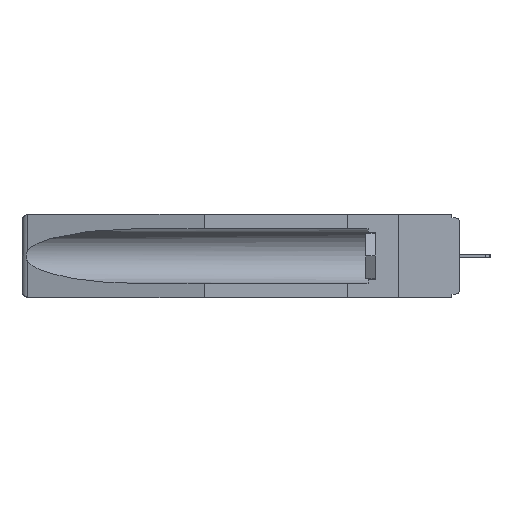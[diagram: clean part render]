
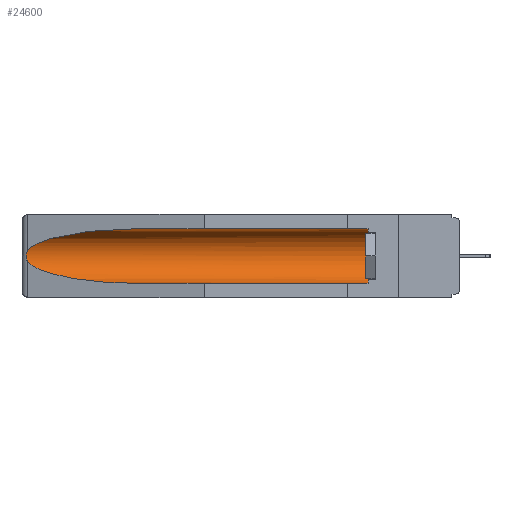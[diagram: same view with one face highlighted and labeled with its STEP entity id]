
A CAD part, left-side view. The second image highlights one B-rep face of the part: STEP entity #24600.
In plain terms, the highlighted cylindrical face has radius 2.857 mm (diameter 5.715 mm), a partial arc.
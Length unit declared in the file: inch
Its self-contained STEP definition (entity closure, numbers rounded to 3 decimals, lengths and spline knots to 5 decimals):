
#1335 = VERTEX_POINT ( 'NONE', #24187 ) ;
#2050 = CARTESIAN_POINT ( 'NONE',  ( 0.155, 1.07973, -0.284 ) ) ;
#2057 = ORIENTED_EDGE ( 'NONE', *, *, #10359, .T. ) ;
#2761 = EDGE_CURVE ( 'NONE', #25303, #18392, #21316, .T. ) ;
#2961 = DIRECTION ( 'NONE',  ( 0., -1., 0. ) ) ;
#3534 = EDGE_CURVE ( 'NONE', #18392, #1335, #25561, .T. ) ;
#4042 = CARTESIAN_POINT ( 'NONE',  ( 0.26597, 1.52961, -0.15275 ) ) ;
#4124 = CARTESIAN_POINT ( 'NONE',  ( 0.21114, 1.30732, -0.284 ) ) ;
#4595 = CARTESIAN_POINT ( 'NONE',  ( 0.2673, 1.53269, -0.17917 ) ) ;
#5179 = CARTESIAN_POINT ( 'NONE',  ( 0.155, 1.07973, -0.059 ) ) ;
#5829 = CYLINDRICAL_SURFACE ( 'NONE', #21166, 0.1125 ) ;
#6156 = CARTESIAN_POINT ( 'NONE',  ( 0.26537, 1.52718, -0.19328 ) ) ;
#6591 = CARTESIAN_POINT ( 'NONE',  ( 0.155, 0.126, -0.284 ) ) ;
#6625 = CARTESIAN_POINT ( 'NONE',  ( 0.26654, 1.53092, -0.15636 ) ) ;
#6821 = CARTESIAN_POINT ( 'NONE',  ( 0.155, -0.30754, -0.284 ) ) ;
#6889 = DIRECTION ( 'NONE',  ( 0., 1., 0. ) ) ;
#7673 = ORIENTED_EDGE ( 'NONE', *, *, #3534, .T. ) ;
#8034 = EDGE_CURVE ( 'NONE', #24053, #15591, #17546, .T. ) ;
#8267 =( BOUNDED_CURVE ( )  B_SPLINE_CURVE ( 3, ( #5179, #26425, #13939, #20240 ),
 .UNSPECIFIED., .F., .T. ) 
 B_SPLINE_CURVE_WITH_KNOTS ( ( 4, 4 ),
 ( 4.71239, 6.08839 ),
 .UNSPECIFIED. ) 
 CURVE ( )  GEOMETRIC_REPRESENTATION_ITEM ( )  RATIONAL_B_SPLINE_CURVE ( ( 1., 0.848, 0.848, 1. ) ) 
 REPRESENTATION_ITEM ( '' )  );
#8889 = CARTESIAN_POINT ( 'NONE',  ( 0.155, 0.126, -0.059 ) ) ;
#10359 = EDGE_CURVE ( 'NONE', #15591, #17185, #16858, .T. ) ;
#10468 = DIRECTION ( 'NONE',  ( 0., 1., 0. ) ) ;
#10754 = CARTESIAN_POINT ( 'NONE',  ( 0.2673, 1.5327, -0.16383 ) ) ;
#10794 = EDGE_CURVE ( 'NONE', #1335, #24053, #8267, .T. ) ;
#11176 = VECTOR ( 'NONE', #22658, 39.37008 ) ;
#11189 = CARTESIAN_POINT ( 'NONE',  ( 0.155, 1.07973, -0.284 ) ) ;
#12402 = CARTESIAN_POINT ( 'NONE',  ( 0.2675, 1.53308, -0.16763 ) ) ;
#12547 = CARTESIAN_POINT ( 'NONE',  ( 0.26537, 1.52718, -0.19328 ) ) ;
#13024 = ORIENTED_EDGE ( 'NONE', *, *, #8034, .T. ) ;
#13166 = CARTESIAN_POINT ( 'NONE',  ( 0.26537, 1.52718, -0.14972 ) ) ;
#13222 = CARTESIAN_POINT ( 'NONE',  ( 0.155, -0.30754, -0.059 ) ) ;
#13298 = EDGE_LOOP ( 'NONE', ( #17951, #13024, #2057, #22222, #24403, #7673 ) ) ;
#13625 = FACE_OUTER_BOUND ( 'NONE', #13298, .T. ) ;
#13939 = CARTESIAN_POINT ( 'NONE',  ( 0.25451, 1.48313, -0.09465 ) ) ;
#14417 = LINE ( 'NONE', #6821, #11176 ) ;
#14547 = CARTESIAN_POINT ( 'NONE',  ( 0.25451, 1.48313, -0.24835 ) ) ;
#15027 = CARTESIAN_POINT ( 'NONE',  ( 0.2675, 1.53308, -0.17534 ) ) ;
#15591 = VERTEX_POINT ( 'NONE', #25670 ) ;
#15660 = AXIS2_PLACEMENT_3D ( 'NONE', #17485, #2961, #21461 ) ;
#16858 =( BOUNDED_CURVE ( )  B_SPLINE_CURVE ( 3, ( #6156, #14547, #4124, #2050 ),
 .UNSPECIFIED., .F., .F. ) 
 B_SPLINE_CURVE_WITH_KNOTS ( ( 4, 4 ),
 ( 0.1948, 1.5708 ),
 .UNSPECIFIED. ) 
 CURVE ( )  GEOMETRIC_REPRESENTATION_ITEM ( )  RATIONAL_B_SPLINE_CURVE ( ( 1., 0.848, 0.848, 1. ) ) 
 REPRESENTATION_ITEM ( '' )  );
#17185 = VERTEX_POINT ( 'NONE', #11189 ) ;
#17485 = CARTESIAN_POINT ( 'NONE',  ( 0.155, 0.126, -0.1715 ) ) ;
#17546 = B_SPLINE_CURVE_WITH_KNOTS ( 'NONE', 3,
 ( #23390, #4042, #6625, #10754, #12402, #15027, #4595, #24894, #20775, #12547 ),
 .UNSPECIFIED., .F., .F.,
 ( 4, 2, 2, 2, 4 ),
 ( 0., 0.00029, 0.00058, 0.00087, 0.00117 ),
 .UNSPECIFIED. ) ;
#17951 = ORIENTED_EDGE ( 'NONE', *, *, #10794, .T. ) ;
#18392 = VERTEX_POINT ( 'NONE', #8889 ) ;
#19733 = VECTOR ( 'NONE', #6889, 39.37008 ) ;
#20240 = CARTESIAN_POINT ( 'NONE',  ( 0.26537, 1.52718, -0.14972 ) ) ;
#20775 = CARTESIAN_POINT ( 'NONE',  ( 0.26597, 1.5296, -0.19026 ) ) ;
#21166 = AXIS2_PLACEMENT_3D ( 'NONE', #22825, #10468, #27075 ) ;
#21316 = CIRCLE ( 'NONE', #15660, 0.1125 ) ;
#21461 = DIRECTION ( 'NONE',  ( 0., 0., 1. ) ) ;
#22222 = ORIENTED_EDGE ( 'NONE', *, *, #22262, .F. ) ;
#22262 = EDGE_CURVE ( 'NONE', #25303, #17185, #14417, .T. ) ;
#22658 = DIRECTION ( 'NONE',  ( 0., 1., 0. ) ) ;
#22825 = CARTESIAN_POINT ( 'NONE',  ( 0.155, -0.30754, -0.1715 ) ) ;
#23390 = CARTESIAN_POINT ( 'NONE',  ( 0.26537, 1.52718, -0.14972 ) ) ;
#24053 = VERTEX_POINT ( 'NONE', #13166 ) ;
#24187 = CARTESIAN_POINT ( 'NONE',  ( 0.155, 1.07973, -0.059 ) ) ;
#24403 = ORIENTED_EDGE ( 'NONE', *, *, #2761, .T. ) ;
#24600 = ADVANCED_FACE ( 'NONE', ( #13625 ), #5829, .F. ) ;
#24894 = CARTESIAN_POINT ( 'NONE',  ( 0.26655, 1.53094, -0.18657 ) ) ;
#25303 = VERTEX_POINT ( 'NONE', #6591 ) ;
#25561 = LINE ( 'NONE', #13222, #19733 ) ;
#25670 = CARTESIAN_POINT ( 'NONE',  ( 0.26537, 1.52718, -0.19328 ) ) ;
#26425 = CARTESIAN_POINT ( 'NONE',  ( 0.21114, 1.30732, -0.059 ) ) ;
#27075 = DIRECTION ( 'NONE',  ( 0., 0., 1. ) ) ;
